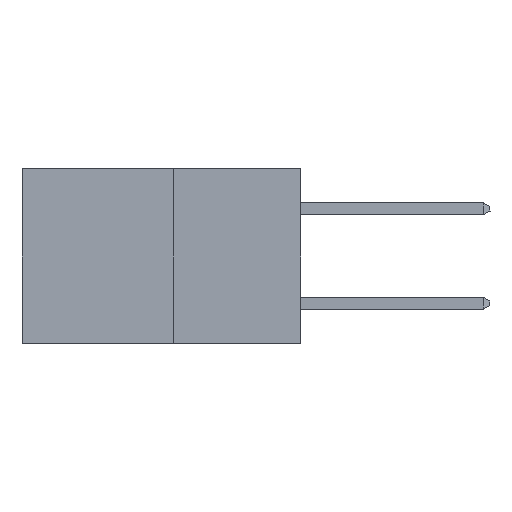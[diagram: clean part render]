
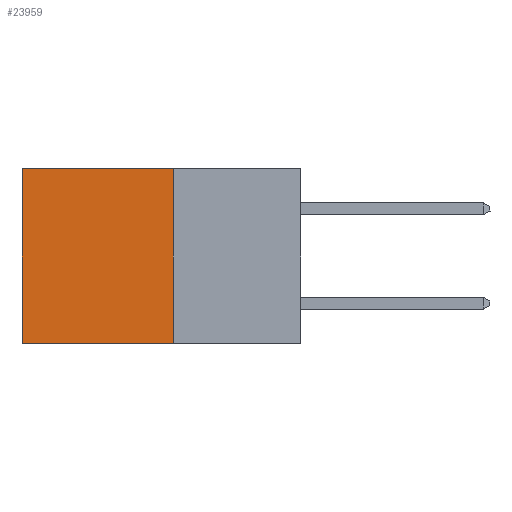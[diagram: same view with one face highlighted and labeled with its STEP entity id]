
A CAD part, left-side view. The second image highlights one B-rep face of the part: STEP entity #23959.
In plain terms, the highlighted planar face has unit normal (-1, 0, 0).
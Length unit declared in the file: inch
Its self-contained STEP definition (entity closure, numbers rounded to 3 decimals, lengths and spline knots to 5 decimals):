
#328 = CARTESIAN_POINT ( 'NONE',  ( 0.277, 0.27, -0.37 ) ) ;
#1763 = VECTOR ( 'NONE', #3004, 39.37008 ) ;
#1929 = CARTESIAN_POINT ( 'NONE',  ( 0.277, 0.27, -0.37 ) ) ;
#2104 = EDGE_LOOP ( 'NONE', ( #18739, #6517, #23348, #4915 ) ) ;
#2603 = LINE ( 'NONE', #328, #1763 ) ;
#3004 = DIRECTION ( 'NONE',  ( 0., 1., 0. ) ) ;
#4562 = VERTEX_POINT ( 'NONE', #30807 ) ;
#4915 = ORIENTED_EDGE ( 'NONE', *, *, #22987, .T. ) ;
#6517 = ORIENTED_EDGE ( 'NONE', *, *, #30569, .F. ) ;
#7594 = FACE_OUTER_BOUND ( 'NONE', #2104, .T. ) ;
#8041 = LINE ( 'NONE', #20144, #20231 ) ;
#8202 = VECTOR ( 'NONE', #22828, 39.37008 ) ;
#8867 = DIRECTION ( 'NONE',  ( 0., 1., 0. ) ) ;
#10099 = VECTOR ( 'NONE', #8867, 39.37008 ) ;
#10176 = VERTEX_POINT ( 'NONE', #10481 ) ;
#10481 = CARTESIAN_POINT ( 'NONE',  ( 0.277, 0.59, 0. ) ) ;
#11617 = EDGE_CURVE ( 'NONE', #10176, #31138, #8041, .T. ) ;
#13316 = CARTESIAN_POINT ( 'NONE',  ( 0.277, 0.59, -0.37 ) ) ;
#13346 = PLANE ( 'NONE',  #25170 ) ;
#15975 = DIRECTION ( 'NONE',  ( 0., 0., -1. ) ) ;
#17836 = LINE ( 'NONE', #29582, #10099 ) ;
#18739 = ORIENTED_EDGE ( 'NONE', *, *, #11617, .T. ) ;
#20144 = CARTESIAN_POINT ( 'NONE',  ( 0.277, 0.59, -0.37 ) ) ;
#20231 = VECTOR ( 'NONE', #33016, 39.37008 ) ;
#22828 = DIRECTION ( 'NONE',  ( 0., 0., -1. ) ) ;
#22987 = EDGE_CURVE ( 'NONE', #4562, #10176, #17836, .T. ) ;
#23348 = ORIENTED_EDGE ( 'NONE', *, *, #33474, .F. ) ;
#23959 = ADVANCED_FACE ( 'NONE', ( #7594 ), #13346, .F. ) ;
#25170 = AXIS2_PLACEMENT_3D ( 'NONE', #31349, #31465, #15975 ) ;
#28258 = VERTEX_POINT ( 'NONE', #31838 ) ;
#28873 = LINE ( 'NONE', #1929, #8202 ) ;
#29582 = CARTESIAN_POINT ( 'NONE',  ( 0.277, 0.27, 0. ) ) ;
#30569 = EDGE_CURVE ( 'NONE', #28258, #31138, #2603, .T. ) ;
#30807 = CARTESIAN_POINT ( 'NONE',  ( 0.277, 0.27, 0. ) ) ;
#31138 = VERTEX_POINT ( 'NONE', #13316 ) ;
#31349 = CARTESIAN_POINT ( 'NONE',  ( 0.277, 0.27, -0.37 ) ) ;
#31465 = DIRECTION ( 'NONE',  ( 1., 0., 0. ) ) ;
#31838 = CARTESIAN_POINT ( 'NONE',  ( 0.277, 0.27, -0.37 ) ) ;
#33016 = DIRECTION ( 'NONE',  ( 0., 0., -1. ) ) ;
#33474 = EDGE_CURVE ( 'NONE', #4562, #28258, #28873, .T. ) ;
